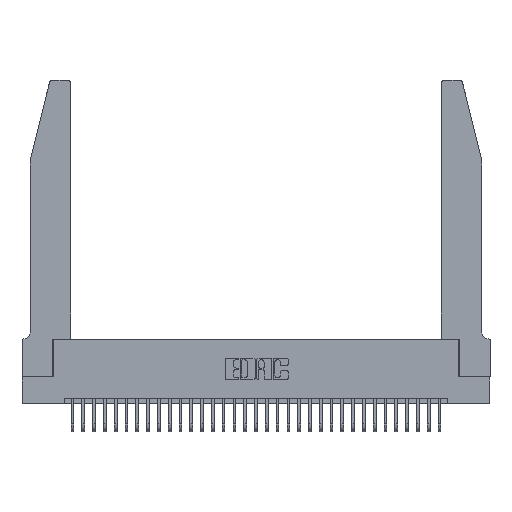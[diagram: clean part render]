
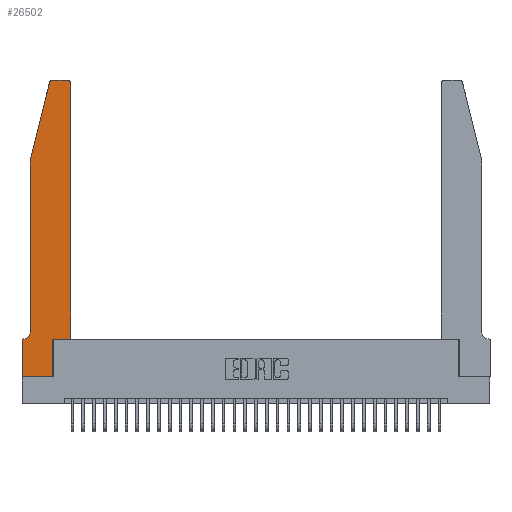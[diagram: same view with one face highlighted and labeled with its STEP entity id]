
A CAD part, top view. The second image highlights one B-rep face of the part: STEP entity #26502.
In plain terms, the highlighted planar face has unit normal (0, 0, 1).
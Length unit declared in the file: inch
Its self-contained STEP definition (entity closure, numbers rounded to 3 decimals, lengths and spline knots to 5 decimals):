
#275 = CARTESIAN_POINT ( 'NONE',  ( 0.2865, 0.35, 0.37 ) ) ;
#626 = CARTESIAN_POINT ( 'NONE',  ( 0.2865, 0., 0.37 ) ) ;
#668 = CARTESIAN_POINT ( 'NONE',  ( 0.4505, 0.35, 0.37 ) ) ;
#952 = VERTEX_POINT ( 'NONE', #20170 ) ;
#1281 = EDGE_CURVE ( 'NONE', #10205, #952, #21865, .T. ) ;
#1284 = CARTESIAN_POINT ( 'NONE',  ( 0., 0., 0.37 ) ) ;
#1390 = ORIENTED_EDGE ( 'NONE', *, *, #6261, .T. ) ;
#1532 = LINE ( 'NONE', #6018, #8235 ) ;
#1964 = ORIENTED_EDGE ( 'NONE', *, *, #11199, .T. ) ;
#2569 = EDGE_CURVE ( 'NONE', #22704, #29572, #13730, .T. ) ;
#2824 = ORIENTED_EDGE ( 'NONE', *, *, #24653, .T. ) ;
#2915 = DIRECTION ( 'NONE',  ( 0., 0., 1. ) ) ;
#3170 = VECTOR ( 'NONE', #15761, 39.37008 ) ;
#3213 = CIRCLE ( 'NONE', #19561, 0.03 ) ;
#3231 = VERTEX_POINT ( 'NONE', #29878 ) ;
#3997 = VECTOR ( 'NONE', #24640, 39.37008 ) ;
#4496 = CIRCLE ( 'NONE', #11343, 0.03 ) ;
#4854 = CARTESIAN_POINT ( 'NONE',  ( 0.2865, 0.35, 0.37 ) ) ;
#5339 = VECTOR ( 'NONE', #28256, 39.37008 ) ;
#5389 = VERTEX_POINT ( 'NONE', #16790 ) ;
#5522 = EDGE_CURVE ( 'NONE', #952, #22657, #29160, .T. ) ;
#5942 = FACE_OUTER_BOUND ( 'NONE', #26619, .T. ) ;
#6018 = CARTESIAN_POINT ( 'NONE',  ( 0.2605, 2.75, 0.37 ) ) ;
#6248 = VECTOR ( 'NONE', #12932, 39.37008 ) ;
#6261 = EDGE_CURVE ( 'NONE', #29572, #25487, #16502, .T. ) ;
#6847 = VECTOR ( 'NONE', #26298, 39.37008 ) ;
#7368 = CARTESIAN_POINT ( 'NONE',  ( 0.4205, 2.72, 0.37 ) ) ;
#8136 = CARTESIAN_POINT ( 'NONE',  ( 0., 0., 0.37 ) ) ;
#8235 = VECTOR ( 'NONE', #20949, 39.37008 ) ;
#8445 = CARTESIAN_POINT ( 'NONE',  ( 0.4505, 2.72, 0.37 ) ) ;
#9296 = VERTEX_POINT ( 'NONE', #24837 ) ;
#9491 = VECTOR ( 'NONE', #15055, 39.37008 ) ;
#9553 = DIRECTION ( 'NONE',  ( 0., 0., -1. ) ) ;
#9560 = ORIENTED_EDGE ( 'NONE', *, *, #22460, .T. ) ;
#9820 = CARTESIAN_POINT ( 'NONE',  ( 0.4505, 0.35, 0.37 ) ) ;
#9910 = DIRECTION ( 'NONE',  ( 1., 0., 0. ) ) ;
#9943 = LINE ( 'NONE', #1284, #22360 ) ;
#10205 = VERTEX_POINT ( 'NONE', #26250 ) ;
#11015 = CARTESIAN_POINT ( 'NONE',  ( 0.0755, 2., 0.37 ) ) ;
#11199 = EDGE_CURVE ( 'NONE', #22657, #22704, #9943, .T. ) ;
#11272 = ORIENTED_EDGE ( 'NONE', *, *, #23921, .T. ) ;
#11343 = AXIS2_PLACEMENT_3D ( 'NONE', #7368, #24734, #9910 ) ;
#12669 = CARTESIAN_POINT ( 'NONE',  ( 0.284, 2.72, 0.37 ) ) ;
#12932 = DIRECTION ( 'NONE',  ( 0., 1., 0. ) ) ;
#13730 = LINE ( 'NONE', #275, #6248 ) ;
#13951 = VERTEX_POINT ( 'NONE', #14819 ) ;
#14469 = EDGE_CURVE ( 'NONE', #25487, #19352, #22290, .T. ) ;
#14554 = EDGE_CURVE ( 'NONE', #9296, #5389, #3213, .T. ) ;
#14819 = CARTESIAN_POINT ( 'NONE',  ( 0.0755, 0.42, 0.37 ) ) ;
#15055 = DIRECTION ( 'NONE',  ( 0., -1., 0. ) ) ;
#15207 = DIRECTION ( 'NONE',  ( 1., 0., 0. ) ) ;
#15341 = VECTOR ( 'NONE', #16506, 39.37008 ) ;
#15407 = EDGE_CURVE ( 'NONE', #15893, #9296, #1532, .T. ) ;
#15761 = DIRECTION ( 'NONE',  ( 1., 0., 0. ) ) ;
#15893 = VERTEX_POINT ( 'NONE', #30537 ) ;
#16086 = AXIS2_PLACEMENT_3D ( 'NONE', #17900, #2915, #20357 ) ;
#16113 = ORIENTED_EDGE ( 'NONE', *, *, #5522, .T. ) ;
#16396 = CARTESIAN_POINT ( 'NONE',  ( 0.0755, 0.35, 0.37 ) ) ;
#16502 = LINE ( 'NONE', #668, #3170 ) ;
#16506 = DIRECTION ( 'NONE',  ( -1., 0., 0. ) ) ;
#16790 = CARTESIAN_POINT ( 'NONE',  ( 0.25487, 2.72718, 0.37 ) ) ;
#17080 = ORIENTED_EDGE ( 'NONE', *, *, #14469, .T. ) ;
#17900 = CARTESIAN_POINT ( 'NONE',  ( 0., 0.35, 0.37 ) ) ;
#18376 = CARTESIAN_POINT ( 'NONE',  ( 0.4505, 0.35, 0.37 ) ) ;
#18716 = CIRCLE ( 'NONE', #31100, 0.07 ) ;
#19352 = VERTEX_POINT ( 'NONE', #8445 ) ;
#19561 = AXIS2_PLACEMENT_3D ( 'NONE', #12669, #29877, #15207 ) ;
#20155 = EDGE_CURVE ( 'NONE', #13951, #10205, #18716, .T. ) ;
#20170 = CARTESIAN_POINT ( 'NONE',  ( 0., 0.35, 0.37 ) ) ;
#20328 = ORIENTED_EDGE ( 'NONE', *, *, #2569, .T. ) ;
#20357 = DIRECTION ( 'NONE',  ( 1., 0., 0. ) ) ;
#20916 = ORIENTED_EDGE ( 'NONE', *, *, #20155, .T. ) ;
#20949 = DIRECTION ( 'NONE',  ( -1., 0., 0. ) ) ;
#21210 = ORIENTED_EDGE ( 'NONE', *, *, #14554, .T. ) ;
#21288 = DIRECTION ( 'NONE',  ( 1., 0., 0. ) ) ;
#21865 = LINE ( 'NONE', #16396, #15341 ) ;
#22290 = LINE ( 'NONE', #9820, #3997 ) ;
#22360 = VECTOR ( 'NONE', #21288, 39.37008 ) ;
#22460 = EDGE_CURVE ( 'NONE', #19352, #15893, #4496, .T. ) ;
#22657 = VERTEX_POINT ( 'NONE', #8136 ) ;
#22704 = VERTEX_POINT ( 'NONE', #626 ) ;
#23625 = LINE ( 'NONE', #11015, #5339 ) ;
#23851 = ORIENTED_EDGE ( 'NONE', *, *, #15407, .T. ) ;
#23864 = CARTESIAN_POINT ( 'NONE',  ( 0.0755, 2., 0.37 ) ) ;
#23921 = EDGE_CURVE ( 'NONE', #3231, #13951, #23625, .T. ) ;
#24390 = CARTESIAN_POINT ( 'NONE',  ( 0.0055, 0.42, 0.37 ) ) ;
#24640 = DIRECTION ( 'NONE',  ( 0., 1., 0. ) ) ;
#24653 = EDGE_CURVE ( 'NONE', #5389, #3231, #26617, .T. ) ;
#24734 = DIRECTION ( 'NONE',  ( 0., 0., 1. ) ) ;
#24837 = CARTESIAN_POINT ( 'NONE',  ( 0.284, 2.75, 0.37 ) ) ;
#25487 = VERTEX_POINT ( 'NONE', #18376 ) ;
#26250 = CARTESIAN_POINT ( 'NONE',  ( 0.0055, 0.35, 0.37 ) ) ;
#26298 = DIRECTION ( 'NONE',  ( -0.239, -0.971, 0. ) ) ;
#26502 = ADVANCED_FACE ( 'NONE', ( #5942 ), #30081, .T. ) ;
#26617 = LINE ( 'NONE', #23864, #6847 ) ;
#26619 = EDGE_LOOP ( 'NONE', ( #23851, #21210, #2824, #11272, #20916, #29690, #16113, #1964, #20328, #1390, #17080, #9560 ) ) ;
#26834 = DIRECTION ( 'NONE',  ( -1., 0., 0. ) ) ;
#26965 = CARTESIAN_POINT ( 'NONE',  ( 0., 0., 0.37 ) ) ;
#28256 = DIRECTION ( 'NONE',  ( 0., -1., 0. ) ) ;
#29160 = LINE ( 'NONE', #26965, #9491 ) ;
#29572 = VERTEX_POINT ( 'NONE', #4854 ) ;
#29690 = ORIENTED_EDGE ( 'NONE', *, *, #1281, .T. ) ;
#29877 = DIRECTION ( 'NONE',  ( 0., 0., 1. ) ) ;
#29878 = CARTESIAN_POINT ( 'NONE',  ( 0.0755, 2., 0.37 ) ) ;
#30081 = PLANE ( 'NONE',  #16086 ) ;
#30537 = CARTESIAN_POINT ( 'NONE',  ( 0.4205, 2.75, 0.37 ) ) ;
#31100 = AXIS2_PLACEMENT_3D ( 'NONE', #24390, #9553, #26834 ) ;
